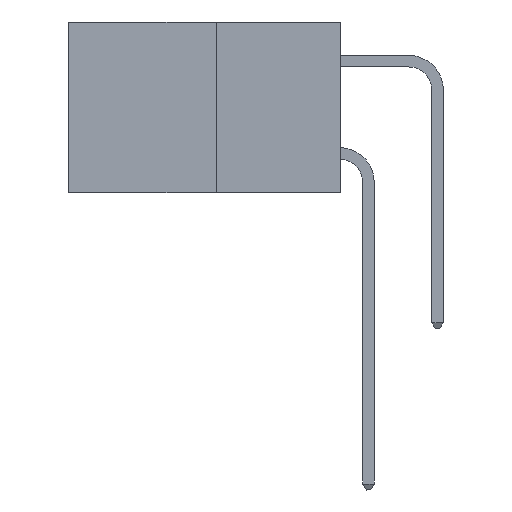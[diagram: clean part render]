
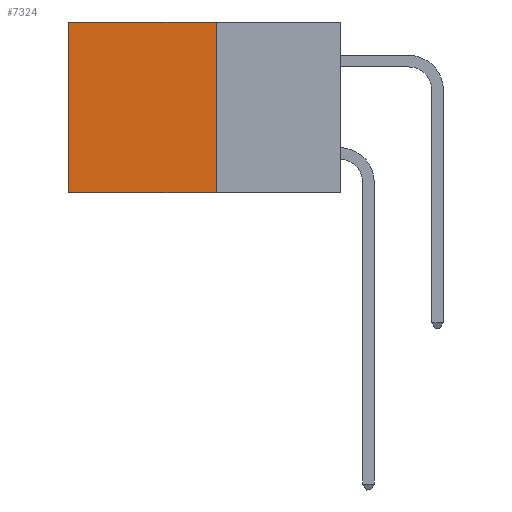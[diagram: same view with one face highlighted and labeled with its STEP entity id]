
A CAD part, left-side view. The second image highlights one B-rep face of the part: STEP entity #7324.
In plain terms, the highlighted planar face has unit normal (-1, 0, 0).
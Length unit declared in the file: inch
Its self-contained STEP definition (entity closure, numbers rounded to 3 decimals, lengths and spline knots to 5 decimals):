
#404 = FACE_OUTER_BOUND ( 'NONE', #7711, .T. ) ;
#475 = CARTESIAN_POINT ( 'NONE',  ( 0.277, 0.27, 0. ) ) ;
#1137 = CARTESIAN_POINT ( 'NONE',  ( 0.277, 0.59, 0. ) ) ;
#1585 = ORIENTED_EDGE ( 'NONE', *, *, #18077, .T. ) ;
#2636 = ORIENTED_EDGE ( 'NONE', *, *, #15316, .F. ) ;
#4180 = VECTOR ( 'NONE', #13594, 39.37008 ) ;
#6777 = DIRECTION ( 'NONE',  ( 0., 1., 0. ) ) ;
#7324 = ADVANCED_FACE ( 'NONE', ( #404 ), #9720, .F. ) ;
#7711 = EDGE_LOOP ( 'NONE', ( #16326, #2636, #18203, #1585 ) ) ;
#8822 = EDGE_CURVE ( 'NONE', #20821, #15767, #16887, .T. ) ;
#9061 = CARTESIAN_POINT ( 'NONE',  ( 0.277, 0.27, -0.37 ) ) ;
#9492 = CARTESIAN_POINT ( 'NONE',  ( 0.277, 0.27, -0.37 ) ) ;
#9720 = PLANE ( 'NONE',  #14673 ) ;
#9964 = EDGE_CURVE ( 'NONE', #15048, #14358, #28297, .T. ) ;
#10315 = CARTESIAN_POINT ( 'NONE',  ( 0.277, 0.59, -0.37 ) ) ;
#10937 = VECTOR ( 'NONE', #28481, 39.37008 ) ;
#11299 = DIRECTION ( 'NONE',  ( 0., 0., -1. ) ) ;
#11689 = DIRECTION ( 'NONE',  ( 1., 0., 0. ) ) ;
#12042 = VECTOR ( 'NONE', #6777, 39.37008 ) ;
#13594 = DIRECTION ( 'NONE',  ( 0., 0., -1. ) ) ;
#13724 = VECTOR ( 'NONE', #18608, 39.37008 ) ;
#14358 = VERTEX_POINT ( 'NONE', #25108 ) ;
#14419 = LINE ( 'NONE', #475, #13724 ) ;
#14673 = AXIS2_PLACEMENT_3D ( 'NONE', #9492, #11689, #11299 ) ;
#15048 = VERTEX_POINT ( 'NONE', #19571 ) ;
#15316 = EDGE_CURVE ( 'NONE', #14358, #15767, #24813, .T. ) ;
#15767 = VERTEX_POINT ( 'NONE', #19430 ) ;
#16326 = ORIENTED_EDGE ( 'NONE', *, *, #8822, .T. ) ;
#16887 = LINE ( 'NONE', #10315, #10937 ) ;
#18077 = EDGE_CURVE ( 'NONE', #15048, #20821, #14419, .T. ) ;
#18203 = ORIENTED_EDGE ( 'NONE', *, *, #9964, .F. ) ;
#18608 = DIRECTION ( 'NONE',  ( 0., 1., 0. ) ) ;
#19430 = CARTESIAN_POINT ( 'NONE',  ( 0.277, 0.59, -0.37 ) ) ;
#19571 = CARTESIAN_POINT ( 'NONE',  ( 0.277, 0.27, 0. ) ) ;
#20821 = VERTEX_POINT ( 'NONE', #1137 ) ;
#24813 = LINE ( 'NONE', #9061, #12042 ) ;
#25108 = CARTESIAN_POINT ( 'NONE',  ( 0.277, 0.27, -0.37 ) ) ;
#27279 = CARTESIAN_POINT ( 'NONE',  ( 0.277, 0.27, -0.37 ) ) ;
#28297 = LINE ( 'NONE', #27279, #4180 ) ;
#28481 = DIRECTION ( 'NONE',  ( 0., 0., -1. ) ) ;
